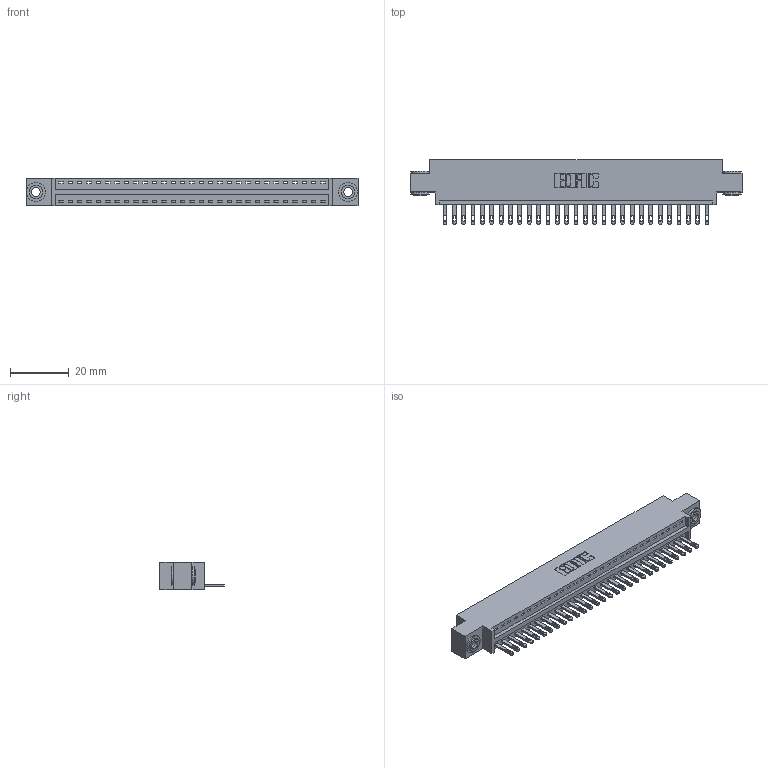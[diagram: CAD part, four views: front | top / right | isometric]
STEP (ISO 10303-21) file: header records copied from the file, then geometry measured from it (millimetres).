
FILE_DESCRIPTION (( 'STEP AP203' ), '1' );
FILE_NAME ('346-029-500-603.STEP', '2022-05-06T08:13:37', ( '' ), ( '' ), 'SwSTEP 2.0', 'SolidWorks 2020', '' );
FILE_SCHEMA (( 'CONFIG_CONTROL_DESIGN' ));
Length unit declared in the file: inch
Products named in the file (4): 345-250-002_345-250-002-102; 346 Part_0.170 Offset - 0.156 Dia-TH; 345-292-001_345-293-100; 346-029-500-603
Assembly tree (32 placements, depth 2):
  346-029-500-603
    346 Part_0.170 Offset - 0.156 Dia-TH
    345-292-001_345-293-100  x29
    345-250-002_345-250-002-102  x2
Bounding box: 112.65 x 21.84 x 9.4 mm (x, y, z)
Volume: 10558.1 mm3; surface area: 13535.3 mm2
Topology: 32 solids, 32 shells, 1744 faces, 5325 edges, 3546 vertices
Faces by surface type: plane 1090, cylinder 646, cone 8
Entity records: 20876 total; most frequent: CARTESIAN_POINT 3564, ORIENTED_EDGE 3518, DIRECTION 3191, EDGE_CURVE 1759, VECTOR 1483, LINE 1483, VERTEX_POINT 1170, AXIS2_PLACEMENT_3D 854
